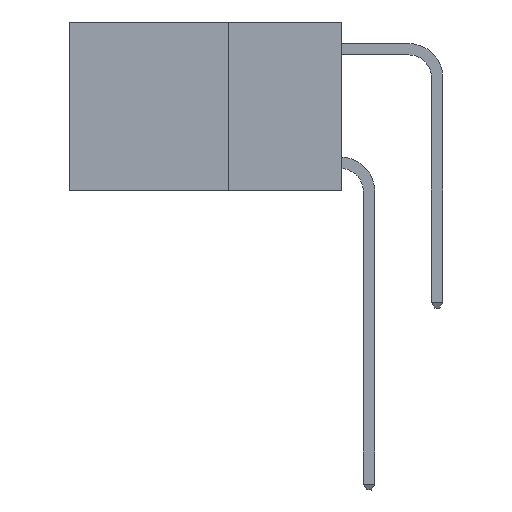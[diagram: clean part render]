
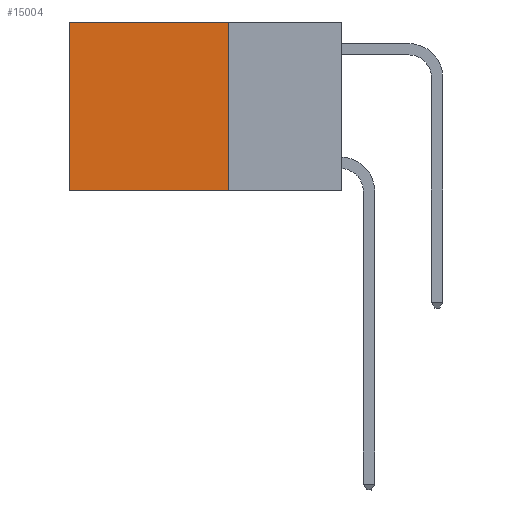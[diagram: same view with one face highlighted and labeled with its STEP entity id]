
A CAD part, left-side view. The second image highlights one B-rep face of the part: STEP entity #15004.
In plain terms, the highlighted planar face has unit normal (-1, 0, 0).
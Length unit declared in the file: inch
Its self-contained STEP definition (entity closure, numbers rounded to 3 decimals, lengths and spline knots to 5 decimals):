
#172 = CARTESIAN_POINT ( 'NONE',  ( 0.2625, 0.25, -0.37 ) ) ;
#543 = LINE ( 'NONE', #20664, #21129 ) ;
#1596 = CARTESIAN_POINT ( 'NONE',  ( 0.2625, 0.25, 0. ) ) ;
#1874 = DIRECTION ( 'NONE',  ( 0., 0., -1. ) ) ;
#2549 = ORIENTED_EDGE ( 'NONE', *, *, #16249, .F. ) ;
#3063 = VECTOR ( 'NONE', #26440, 39.37008 ) ;
#3608 = VERTEX_POINT ( 'NONE', #19481 ) ;
#5051 = AXIS2_PLACEMENT_3D ( 'NONE', #1596, #17035, #9517 ) ;
#6678 = VECTOR ( 'NONE', #17700, 39.37008 ) ;
#7735 = EDGE_CURVE ( 'NONE', #19175, #3608, #29664, .T. ) ;
#7804 = CARTESIAN_POINT ( 'NONE',  ( 0.2625, 0.25, -0.37 ) ) ;
#8187 = ORIENTED_EDGE ( 'NONE', *, *, #7735, .T. ) ;
#9517 = DIRECTION ( 'NONE',  ( 0., 0., -1. ) ) ;
#9960 = LINE ( 'NONE', #172, #3063 ) ;
#9975 = FACE_OUTER_BOUND ( 'NONE', #29147, .T. ) ;
#15004 = ADVANCED_FACE ( 'NONE', ( #9975 ), #19758, .F. ) ;
#15815 = VERTEX_POINT ( 'NONE', #28330 ) ;
#16212 = LINE ( 'NONE', #25459, #24279 ) ;
#16241 = ORIENTED_EDGE ( 'NONE', *, *, #17439, .T. ) ;
#16249 = EDGE_CURVE ( 'NONE', #19175, #31237, #543, .T. ) ;
#17035 = DIRECTION ( 'NONE',  ( 1., 0., 0. ) ) ;
#17439 = EDGE_CURVE ( 'NONE', #3608, #15815, #16212, .T. ) ;
#17700 = DIRECTION ( 'NONE',  ( 0., 1., 0. ) ) ;
#19175 = VERTEX_POINT ( 'NONE', #28623 ) ;
#19481 = CARTESIAN_POINT ( 'NONE',  ( 0.2625, 0.6, 0. ) ) ;
#19758 = PLANE ( 'NONE',  #5051 ) ;
#20619 = CARTESIAN_POINT ( 'NONE',  ( 0.2625, 0.25, 0. ) ) ;
#20664 = CARTESIAN_POINT ( 'NONE',  ( 0.2625, 0.25, 0. ) ) ;
#21129 = VECTOR ( 'NONE', #28321, 39.37008 ) ;
#24279 = VECTOR ( 'NONE', #1874, 39.37008 ) ;
#25459 = CARTESIAN_POINT ( 'NONE',  ( 0.2625, 0.6, 0. ) ) ;
#26440 = DIRECTION ( 'NONE',  ( 0., 1., 0. ) ) ;
#28321 = DIRECTION ( 'NONE',  ( 0., 0., -1. ) ) ;
#28330 = CARTESIAN_POINT ( 'NONE',  ( 0.2625, 0.6, -0.37 ) ) ;
#28623 = CARTESIAN_POINT ( 'NONE',  ( 0.2625, 0.25, 0. ) ) ;
#28689 = ORIENTED_EDGE ( 'NONE', *, *, #32488, .F. ) ;
#29147 = EDGE_LOOP ( 'NONE', ( #16241, #28689, #2549, #8187 ) ) ;
#29664 = LINE ( 'NONE', #20619, #6678 ) ;
#31237 = VERTEX_POINT ( 'NONE', #7804 ) ;
#32488 = EDGE_CURVE ( 'NONE', #31237, #15815, #9960, .T. ) ;
